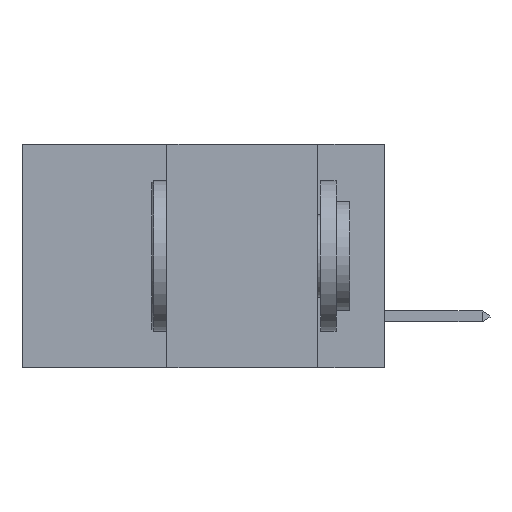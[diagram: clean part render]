
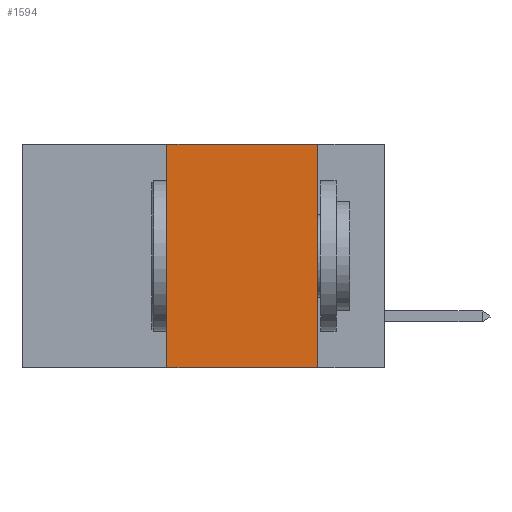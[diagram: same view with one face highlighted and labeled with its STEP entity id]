
A CAD part, left-side view. The second image highlights one B-rep face of the part: STEP entity #1594.
In plain terms, the highlighted planar face has unit normal (-1, 0, 0).
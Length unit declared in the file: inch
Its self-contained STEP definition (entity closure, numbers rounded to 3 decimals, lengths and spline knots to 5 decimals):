
#58 = CARTESIAN_POINT ( 'NONE',  ( 0., 0.36, 0. ) ) ;
#1151 = ORIENTED_EDGE ( 'NONE', *, *, #3556, .F. ) ;
#1217 = VERTEX_POINT ( 'NONE', #58 ) ;
#1559 = VECTOR ( 'NONE', #8523, 39.37008 ) ;
#1594 = ADVANCED_FACE ( 'NONE', ( #3646 ), #1722, .F. ) ;
#1613 = DIRECTION ( 'NONE',  ( 0., 0., -1. ) ) ;
#1631 = DIRECTION ( 'NONE',  ( 1., 0., 0. ) ) ;
#1722 = PLANE ( 'NONE',  #3152 ) ;
#2661 = VECTOR ( 'NONE', #10235, 39.37008 ) ;
#2662 = CARTESIAN_POINT ( 'NONE',  ( 0., 0.6, 0. ) ) ;
#2820 = EDGE_CURVE ( 'NONE', #7252, #7424, #4003, .T. ) ;
#3152 = AXIS2_PLACEMENT_3D ( 'NONE', #2662, #1631, #1613 ) ;
#3333 = LINE ( 'NONE', #8319, #7600 ) ;
#3356 = EDGE_CURVE ( 'NONE', #1217, #7252, #9428, .T. ) ;
#3427 = ORIENTED_EDGE ( 'NONE', *, *, #2820, .F. ) ;
#3556 = EDGE_CURVE ( 'NONE', #10921, #1217, #3333, .T. ) ;
#3646 = FACE_OUTER_BOUND ( 'NONE', #5889, .T. ) ;
#4003 = LINE ( 'NONE', #9299, #1559 ) ;
#4293 = CARTESIAN_POINT ( 'NONE',  ( 0., 0.11, 0. ) ) ;
#4761 = VECTOR ( 'NONE', #7684, 39.37008 ) ;
#5355 = CARTESIAN_POINT ( 'NONE',  ( 0., 0.36, -0.37 ) ) ;
#5775 = EDGE_CURVE ( 'NONE', #10921, #7424, #7032, .T. ) ;
#5889 = EDGE_LOOP ( 'NONE', ( #3427, #7956, #1151, #5930 ) ) ;
#5930 = ORIENTED_EDGE ( 'NONE', *, *, #5775, .T. ) ;
#6328 = CARTESIAN_POINT ( 'NONE',  ( 0., 0.6, -0.37 ) ) ;
#7032 = LINE ( 'NONE', #6328, #4761 ) ;
#7252 = VERTEX_POINT ( 'NONE', #4293 ) ;
#7424 = VERTEX_POINT ( 'NONE', #9595 ) ;
#7600 = VECTOR ( 'NONE', #9733, 39.37008 ) ;
#7684 = DIRECTION ( 'NONE',  ( 0., -1., 0. ) ) ;
#7956 = ORIENTED_EDGE ( 'NONE', *, *, #3356, .F. ) ;
#8319 = CARTESIAN_POINT ( 'NONE',  ( 0., 0.36, 0. ) ) ;
#8523 = DIRECTION ( 'NONE',  ( 0., 0., -1. ) ) ;
#9299 = CARTESIAN_POINT ( 'NONE',  ( 0., 0.11, 0. ) ) ;
#9428 = LINE ( 'NONE', #10158, #2661 ) ;
#9595 = CARTESIAN_POINT ( 'NONE',  ( 0., 0.11, -0.37 ) ) ;
#9733 = DIRECTION ( 'NONE',  ( 0., 0., 1. ) ) ;
#10158 = CARTESIAN_POINT ( 'NONE',  ( 0., 0.6, 0. ) ) ;
#10235 = DIRECTION ( 'NONE',  ( 0., -1., 0. ) ) ;
#10921 = VERTEX_POINT ( 'NONE', #5355 ) ;
